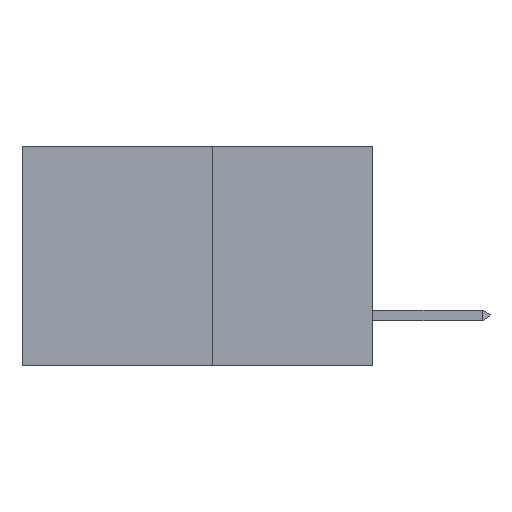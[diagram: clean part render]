
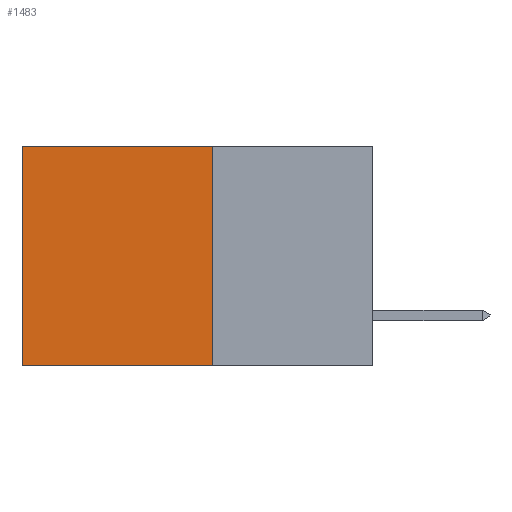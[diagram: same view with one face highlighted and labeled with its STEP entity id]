
A CAD part, left-side view. The second image highlights one B-rep face of the part: STEP entity #1483.
In plain terms, the highlighted planar face has unit normal (-1, 0, 0).
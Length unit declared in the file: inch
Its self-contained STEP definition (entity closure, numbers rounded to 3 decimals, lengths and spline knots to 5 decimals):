
#1102 = CARTESIAN_POINT ( 'NONE',  ( 0.277, 0.27, 0. ) ) ;
#1483 = ADVANCED_FACE ( 'NONE', ( #20038 ), #28571, .F. ) ;
#1591 = EDGE_LOOP ( 'NONE', ( #2671, #24752, #10112, #25845 ) ) ;
#2671 = ORIENTED_EDGE ( 'NONE', *, *, #14792, .T. ) ;
#2721 = DIRECTION ( 'NONE',  ( 1., 0., 0. ) ) ;
#2810 = CARTESIAN_POINT ( 'NONE',  ( 0.277, 0.27, -0.37 ) ) ;
#2830 = CARTESIAN_POINT ( 'NONE',  ( 0.277, 0.27, -0.37 ) ) ;
#3390 = VERTEX_POINT ( 'NONE', #8184 ) ;
#4985 = DIRECTION ( 'NONE',  ( 0., 1., 0. ) ) ;
#6218 = AXIS2_PLACEMENT_3D ( 'NONE', #2810, #2721, #15209 ) ;
#6230 = CARTESIAN_POINT ( 'NONE',  ( 0.277, 0.59, -0.37 ) ) ;
#6460 = VERTEX_POINT ( 'NONE', #8138 ) ;
#7726 = LINE ( 'NONE', #6230, #19789 ) ;
#8138 = CARTESIAN_POINT ( 'NONE',  ( 0.277, 0.59, 0. ) ) ;
#8184 = CARTESIAN_POINT ( 'NONE',  ( 0.277, 0.27, -0.37 ) ) ;
#8694 = DIRECTION ( 'NONE',  ( 0., 0., -1. ) ) ;
#9303 = VECTOR ( 'NONE', #28728, 39.37008 ) ;
#10112 = ORIENTED_EDGE ( 'NONE', *, *, #26227, .F. ) ;
#14792 = EDGE_CURVE ( 'NONE', #6460, #22713, #7726, .T. ) ;
#15209 = DIRECTION ( 'NONE',  ( 0., 0., -1. ) ) ;
#15374 = VERTEX_POINT ( 'NONE', #1102 ) ;
#15431 = CARTESIAN_POINT ( 'NONE',  ( 0.277, 0.59, -0.37 ) ) ;
#16988 = CARTESIAN_POINT ( 'NONE',  ( 0.277, 0.27, 0. ) ) ;
#17475 = EDGE_CURVE ( 'NONE', #15374, #6460, #27915, .T. ) ;
#17770 = DIRECTION ( 'NONE',  ( 0., 1., 0. ) ) ;
#19789 = VECTOR ( 'NONE', #8694, 39.37008 ) ;
#20038 = FACE_OUTER_BOUND ( 'NONE', #1591, .T. ) ;
#22310 = VECTOR ( 'NONE', #17770, 39.37008 ) ;
#22713 = VERTEX_POINT ( 'NONE', #15431 ) ;
#24752 = ORIENTED_EDGE ( 'NONE', *, *, #30316, .F. ) ;
#25845 = ORIENTED_EDGE ( 'NONE', *, *, #17475, .T. ) ;
#26227 = EDGE_CURVE ( 'NONE', #15374, #3390, #29295, .T. ) ;
#27172 = VECTOR ( 'NONE', #4985, 39.37008 ) ;
#27915 = LINE ( 'NONE', #16988, #27172 ) ;
#28571 = PLANE ( 'NONE',  #6218 ) ;
#28689 = LINE ( 'NONE', #2830, #22310 ) ;
#28728 = DIRECTION ( 'NONE',  ( 0., 0., -1. ) ) ;
#29209 = CARTESIAN_POINT ( 'NONE',  ( 0.277, 0.27, -0.37 ) ) ;
#29295 = LINE ( 'NONE', #29209, #9303 ) ;
#30316 = EDGE_CURVE ( 'NONE', #3390, #22713, #28689, .T. ) ;
